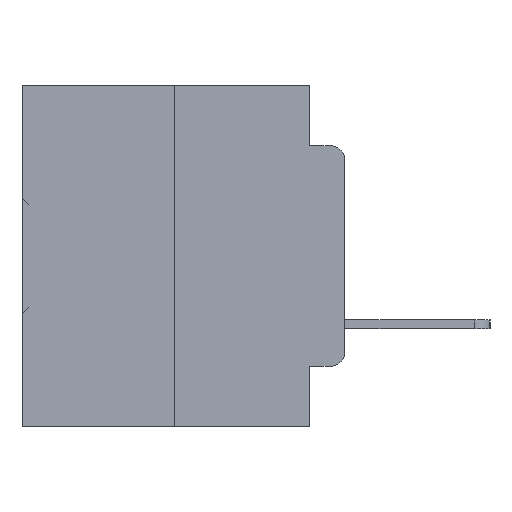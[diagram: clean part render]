
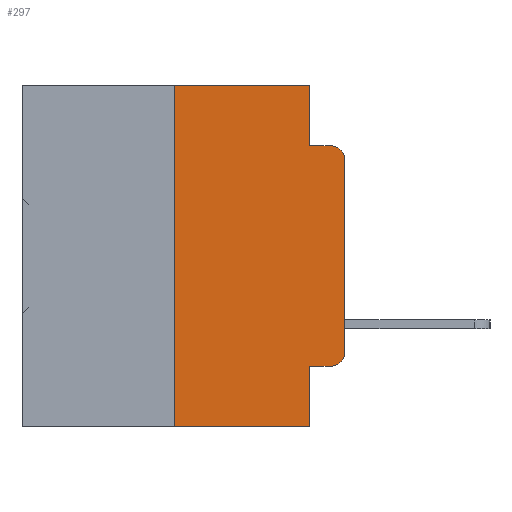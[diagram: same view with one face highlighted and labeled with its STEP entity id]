
A CAD part, left-side view. The second image highlights one B-rep face of the part: STEP entity #297.
In plain terms, the highlighted planar face has unit normal (-1, 0, 0).
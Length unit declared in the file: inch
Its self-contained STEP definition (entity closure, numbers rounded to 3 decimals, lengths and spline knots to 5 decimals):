
#297 = ADVANCED_FACE ( 'NONE', ( #15529 ), #14344, .F. ) ;
#624 = LINE ( 'NONE', #20810, #23117 ) ;
#1822 = CARTESIAN_POINT ( 'NONE',  ( 0., 0.473, 0. ) ) ;
#1898 = ORIENTED_EDGE ( 'NONE', *, *, #17008, .T. ) ;
#2855 = VERTEX_POINT ( 'NONE', #12935 ) ;
#3029 = EDGE_CURVE ( 'NONE', #3897, #3609, #624, .T. ) ;
#3609 = VERTEX_POINT ( 'NONE', #35670 ) ;
#3897 = VERTEX_POINT ( 'NONE', #34949 ) ;
#4314 = LINE ( 'NONE', #32410, #20187 ) ;
#4944 = VERTEX_POINT ( 'NONE', #18456 ) ;
#5492 = EDGE_CURVE ( 'NONE', #25679, #21782, #29889, .T. ) ;
#6075 = CARTESIAN_POINT ( 'NONE',  ( 0., 0., 0. ) ) ;
#6976 = EDGE_LOOP ( 'NONE', ( #11332, #25970, #26821, #22157, #23870, #11777, #33611, #35271, #1898, #26008 ) ) ;
#7805 = LINE ( 'NONE', #13653, #21794 ) ;
#7855 = DIRECTION ( 'NONE',  ( 0., 0., -1. ) ) ;
#8992 = EDGE_CURVE ( 'NONE', #21782, #9121, #21161, .T. ) ;
#9121 = VERTEX_POINT ( 'NONE', #30567 ) ;
#9658 = AXIS2_PLACEMENT_3D ( 'NONE', #30390, #14000, #33096 ) ;
#9885 = LINE ( 'NONE', #14992, #31815 ) ;
#10475 = AXIS2_PLACEMENT_3D ( 'NONE', #16398, #35367, #19176 ) ;
#10622 = DIRECTION ( 'NONE',  ( 0., 0., -1. ) ) ;
#11332 = ORIENTED_EDGE ( 'NONE', *, *, #5492, .T. ) ;
#11777 = ORIENTED_EDGE ( 'NONE', *, *, #27060, .F. ) ;
#12483 = CARTESIAN_POINT ( 'NONE',  ( 0., 0.02, -0.4115 ) ) ;
#12935 = CARTESIAN_POINT ( 'NONE',  ( 0., 0.051, -0.0885 ) ) ;
#13078 = VERTEX_POINT ( 'NONE', #18319 ) ;
#13286 = DIRECTION ( 'NONE',  ( 0., -1., 0. ) ) ;
#13653 = CARTESIAN_POINT ( 'NONE',  ( 0., 0.25, 0. ) ) ;
#14000 = DIRECTION ( 'NONE',  ( -1., 0., 0. ) ) ;
#14344 = PLANE ( 'NONE',  #31489 ) ;
#14992 = CARTESIAN_POINT ( 'NONE',  ( 0., 0.051, -0.0885 ) ) ;
#15370 = VECTOR ( 'NONE', #27673, 39.37008 ) ;
#15529 = FACE_OUTER_BOUND ( 'NONE', #6976, .T. ) ;
#15684 = DIRECTION ( 'NONE',  ( 0., 0., -1. ) ) ;
#16398 = CARTESIAN_POINT ( 'NONE',  ( 0., 0.02, -0.1085 ) ) ;
#17008 = EDGE_CURVE ( 'NONE', #4944, #31293, #4314, .T. ) ;
#18049 = CARTESIAN_POINT ( 'NONE',  ( 0., 0., -0.1085 ) ) ;
#18167 = CIRCLE ( 'NONE', #9658, 0.02 ) ;
#18319 = CARTESIAN_POINT ( 'NONE',  ( 0., 0.051, 0. ) ) ;
#18456 = CARTESIAN_POINT ( 'NONE',  ( 0., 0.051, -0.4115 ) ) ;
#18810 = DIRECTION ( 'NONE',  ( 1., 0., 0. ) ) ;
#19176 = DIRECTION ( 'NONE',  ( 0., 0., -1. ) ) ;
#19377 = LINE ( 'NONE', #29280, #33795 ) ;
#20004 = EDGE_CURVE ( 'NONE', #4944, #3609, #19377, .T. ) ;
#20187 = VECTOR ( 'NONE', #13286, 39.37008 ) ;
#20810 = CARTESIAN_POINT ( 'NONE',  ( 0., 0.473, -0.5 ) ) ;
#21161 = CIRCLE ( 'NONE', #10475, 0.02 ) ;
#21782 = VERTEX_POINT ( 'NONE', #18049 ) ;
#21794 = VECTOR ( 'NONE', #30056, 39.37008 ) ;
#22157 = ORIENTED_EDGE ( 'NONE', *, *, #34309, .F. ) ;
#22405 = VECTOR ( 'NONE', #30199, 39.37008 ) ;
#23117 = VECTOR ( 'NONE', #29121, 39.37008 ) ;
#23870 = ORIENTED_EDGE ( 'NONE', *, *, #34364, .F. ) ;
#24097 = VECTOR ( 'NONE', #7855, 39.37008 ) ;
#24313 = EDGE_CURVE ( 'NONE', #31293, #25679, #18167, .T. ) ;
#24949 = LINE ( 'NONE', #29967, #24097 ) ;
#25679 = VERTEX_POINT ( 'NONE', #32187 ) ;
#25970 = ORIENTED_EDGE ( 'NONE', *, *, #8992, .T. ) ;
#26008 = ORIENTED_EDGE ( 'NONE', *, *, #24313, .T. ) ;
#26642 = VERTEX_POINT ( 'NONE', #28311 ) ;
#26821 = ORIENTED_EDGE ( 'NONE', *, *, #32970, .F. ) ;
#27060 = EDGE_CURVE ( 'NONE', #3897, #26642, #7805, .T. ) ;
#27485 = CARTESIAN_POINT ( 'NONE',  ( 0., 0.473, 0. ) ) ;
#27673 = DIRECTION ( 'NONE',  ( 0., 0., 1. ) ) ;
#28311 = CARTESIAN_POINT ( 'NONE',  ( 0., 0.25, 0. ) ) ;
#29121 = DIRECTION ( 'NONE',  ( 0., -1., 0. ) ) ;
#29280 = CARTESIAN_POINT ( 'NONE',  ( 0., 0.051, 0. ) ) ;
#29596 = LINE ( 'NONE', #27485, #22405 ) ;
#29889 = LINE ( 'NONE', #6075, #15370 ) ;
#29967 = CARTESIAN_POINT ( 'NONE',  ( 0., 0.051, 0. ) ) ;
#30056 = DIRECTION ( 'NONE',  ( 0., 0., 1. ) ) ;
#30199 = DIRECTION ( 'NONE',  ( 0., -1., 0. ) ) ;
#30390 = CARTESIAN_POINT ( 'NONE',  ( 0., 0.02, -0.3915 ) ) ;
#30567 = CARTESIAN_POINT ( 'NONE',  ( 0., 0.02, -0.0885 ) ) ;
#31293 = VERTEX_POINT ( 'NONE', #12483 ) ;
#31489 = AXIS2_PLACEMENT_3D ( 'NONE', #1822, #18810, #10622 ) ;
#31815 = VECTOR ( 'NONE', #34043, 39.37008 ) ;
#32187 = CARTESIAN_POINT ( 'NONE',  ( 0., 0., -0.3915 ) ) ;
#32410 = CARTESIAN_POINT ( 'NONE',  ( 0., 0.051, -0.4115 ) ) ;
#32970 = EDGE_CURVE ( 'NONE', #2855, #9121, #9885, .T. ) ;
#33096 = DIRECTION ( 'NONE',  ( 0., 0., -1. ) ) ;
#33611 = ORIENTED_EDGE ( 'NONE', *, *, #3029, .T. ) ;
#33795 = VECTOR ( 'NONE', #15684, 39.37008 ) ;
#34043 = DIRECTION ( 'NONE',  ( 0., -1., 0. ) ) ;
#34309 = EDGE_CURVE ( 'NONE', #13078, #2855, #24949, .T. ) ;
#34364 = EDGE_CURVE ( 'NONE', #26642, #13078, #29596, .T. ) ;
#34949 = CARTESIAN_POINT ( 'NONE',  ( 0., 0.25, -0.5 ) ) ;
#35271 = ORIENTED_EDGE ( 'NONE', *, *, #20004, .F. ) ;
#35367 = DIRECTION ( 'NONE',  ( -1., 0., 0. ) ) ;
#35670 = CARTESIAN_POINT ( 'NONE',  ( 0., 0.051, -0.5 ) ) ;
